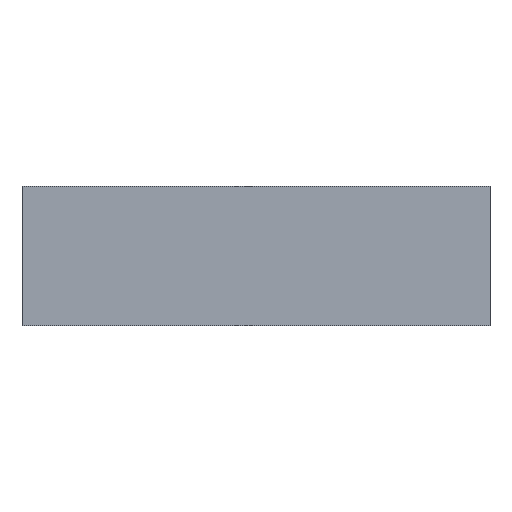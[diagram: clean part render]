
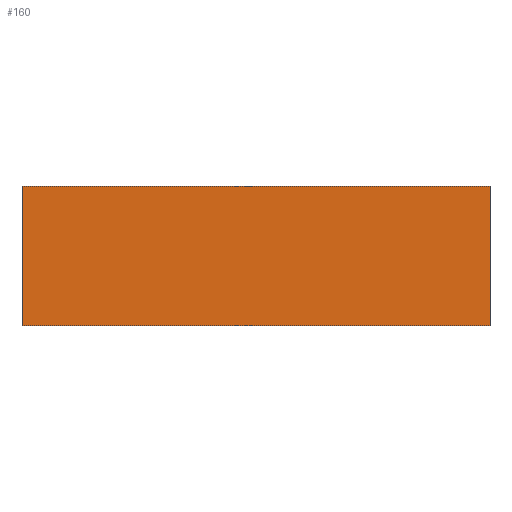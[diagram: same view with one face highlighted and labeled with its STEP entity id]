
A CAD part, front view. The second image highlights one B-rep face of the part: STEP entity #160.
In plain terms, the highlighted planar face has unit normal (0, -1, 0).
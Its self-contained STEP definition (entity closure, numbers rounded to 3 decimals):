
#12 = ORIENTED_EDGE ( 'NONE', *, *, #1136, .F. ) ;
#17 = ORIENTED_EDGE ( 'NONE', *, *, #1038, .T. ) ;
#53 = VERTEX_POINT ( 'NONE', #1376 ) ;
#127 = VECTOR ( 'NONE', #1274, 1000. ) ;
#160 = ADVANCED_FACE ( 'NONE', ( #390 ), #902, .F. ) ;
#325 = CARTESIAN_POINT ( 'NONE',  ( -25.2, -50.325, 0. ) ) ;
#326 = CARTESIAN_POINT ( 'NONE',  ( -25.2, -50.325, 15. ) ) ;
#334 = CARTESIAN_POINT ( 'NONE',  ( 25.2, -50.325, 15. ) ) ;
#341 = VERTEX_POINT ( 'NONE', #821 ) ;
#372 = ORIENTED_EDGE ( 'NONE', *, *, #1246, .F. ) ;
#390 = FACE_OUTER_BOUND ( 'NONE', #416, .T. ) ;
#416 = EDGE_LOOP ( 'NONE', ( #17, #12, #372, #1378 ) ) ;
#445 = DIRECTION ( 'NONE',  ( 0., 0., -1. ) ) ;
#446 = LINE ( 'NONE', #1290, #127 ) ;
#462 = DIRECTION ( 'NONE',  ( 1., 0., 0. ) ) ;
#514 = CARTESIAN_POINT ( 'NONE',  ( -25.2, -50.325, 0. ) ) ;
#559 = VECTOR ( 'NONE', #1080, 1000. ) ;
#597 = LINE ( 'NONE', #1427, #1108 ) ;
#735 = CARTESIAN_POINT ( 'NONE',  ( -25.2, -50.325, 15. ) ) ;
#747 = VERTEX_POINT ( 'NONE', #514 ) ;
#777 = AXIS2_PLACEMENT_3D ( 'NONE', #326, #1155, #1243 ) ;
#796 = VECTOR ( 'NONE', #445, 1000. ) ;
#821 = CARTESIAN_POINT ( 'NONE',  ( 25.2, -50.325, 15. ) ) ;
#900 = LINE ( 'NONE', #334, #796 ) ;
#902 = PLANE ( 'NONE',  #777 ) ;
#1038 = EDGE_CURVE ( 'NONE', #747, #53, #1195, .T. ) ;
#1070 = EDGE_CURVE ( 'NONE', #1502, #747, #446, .T. ) ;
#1080 = DIRECTION ( 'NONE',  ( 1., 0., 0. ) ) ;
#1108 = VECTOR ( 'NONE', #462, 1000. ) ;
#1136 = EDGE_CURVE ( 'NONE', #341, #53, #900, .T. ) ;
#1155 = DIRECTION ( 'NONE',  ( 0., 1., 0. ) ) ;
#1195 = LINE ( 'NONE', #325, #559 ) ;
#1243 = DIRECTION ( 'NONE',  ( 0., 0., 1. ) ) ;
#1246 = EDGE_CURVE ( 'NONE', #1502, #341, #597, .T. ) ;
#1274 = DIRECTION ( 'NONE',  ( 0., 0., -1. ) ) ;
#1290 = CARTESIAN_POINT ( 'NONE',  ( -25.2, -50.325, 15. ) ) ;
#1376 = CARTESIAN_POINT ( 'NONE',  ( 25.2, -50.325, 0. ) ) ;
#1378 = ORIENTED_EDGE ( 'NONE', *, *, #1070, .T. ) ;
#1427 = CARTESIAN_POINT ( 'NONE',  ( -25.2, -50.325, 15. ) ) ;
#1502 = VERTEX_POINT ( 'NONE', #735 ) ;
